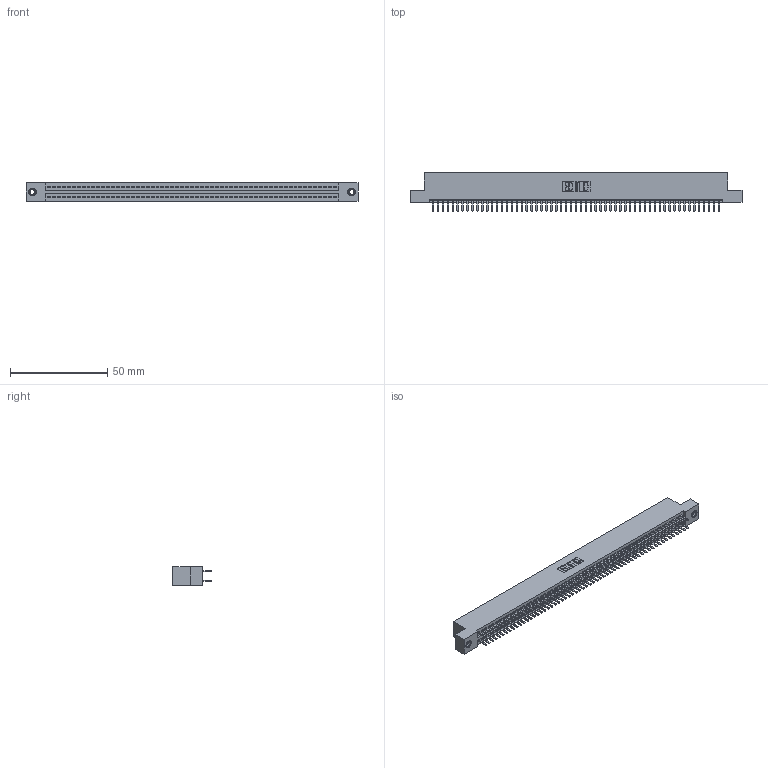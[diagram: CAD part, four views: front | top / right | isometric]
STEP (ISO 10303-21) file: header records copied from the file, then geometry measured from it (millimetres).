
FILE_DESCRIPTION (( 'STEP AP203' ), '1' );
FILE_NAME ('395-118-520-207.STEP', '2018-12-02T04:28:54', ( '' ), ( '' ), 'SwSTEP 2.0', 'SolidWorks 2016', '' );
FILE_SCHEMA (( 'CONFIG_CONTROL_DESIGN' ));
Length unit declared in the file: inch
Products named in the file (4): 395-118-520-207; 345 Part_Flush Mounting Lugs - 0.156 Dia-TI; 345-250-001_345-250-005-103; 345-292-001_345-293-120
Assembly tree (121 placements, depth 2):
  395-118-520-207
    345 Part_Flush Mounting Lugs - 0.156 Dia-TI
    345-292-001_345-293-120  x118
    345-250-001_345-250-005-103  x2
Bounding box: 171.07 x 19.68 x 9.4 mm (x, y, z)
Volume: 16710.2 mm3; surface area: 24947.3 mm2
Topology: 121 solids, 121 shells, 6558 faces, 19003 edges, 12346 vertices
Faces by surface type: plane 4242, cylinder 2300, cone 12, torus 4
Entity records: 45304 total; most frequent: CARTESIAN_POINT 7571, ORIENTED_EDGE 7486, DIRECTION 6669, EDGE_CURVE 3743, LINE 3351, VECTOR 3351, VERTEX_POINT 2488, AXIS2_PLACEMENT_3D 1659
